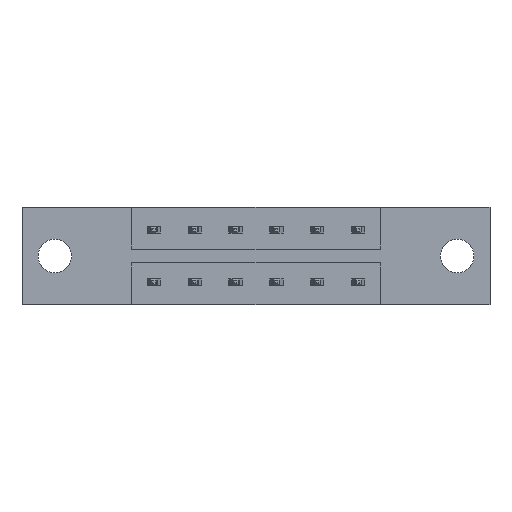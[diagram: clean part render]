
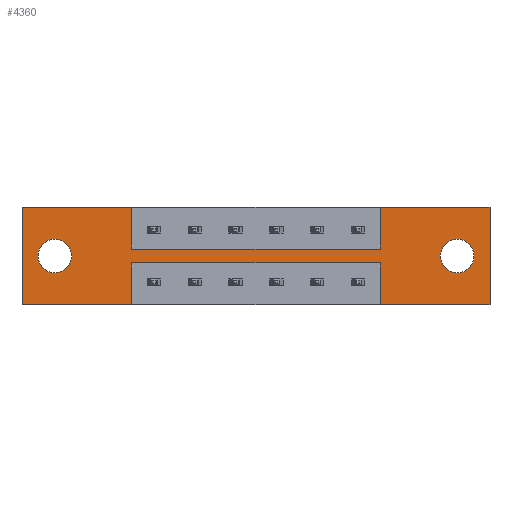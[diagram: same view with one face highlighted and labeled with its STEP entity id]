
A CAD part, front view. The second image highlights one B-rep face of the part: STEP entity #4360.
In plain terms, the highlighted planar face has unit normal (0, -1, 0).
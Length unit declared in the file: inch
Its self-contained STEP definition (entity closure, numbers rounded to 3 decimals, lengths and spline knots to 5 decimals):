
#83 = DIRECTION ( 'NONE',  ( 0., 0., 1. ) ) ;
#86 = EDGE_CURVE ( 'NONE', #4618, #5407, #849, .T. ) ;
#209 = DIRECTION ( 'NONE',  ( 0., 1., 0. ) ) ;
#345 = LINE ( 'NONE', #2995, #7201 ) ;
#614 = DIRECTION ( 'NONE',  ( 0., 1., 0. ) ) ;
#626 = CARTESIAN_POINT ( 'NONE',  ( 0., 0., -0.37 ) ) ;
#818 = EDGE_CURVE ( 'NONE', #3925, #4857, #345, .T. ) ;
#849 = CIRCLE ( 'NONE', #7057, 0.064 ) ;
#863 = EDGE_CURVE ( 'NONE', #5407, #4618, #3503, .T. ) ;
#880 = CIRCLE ( 'NONE', #7218, 0.064 ) ;
#951 = ORIENTED_EDGE ( 'NONE', *, *, #6117, .F. ) ;
#955 = FACE_OUTER_BOUND ( 'NONE', #8546, .T. ) ;
#981 = CARTESIAN_POINT ( 'NONE',  ( 1.3665, 0., -0.1585 ) ) ;
#999 = CARTESIAN_POINT ( 'NONE',  ( 1.659, 0., -0.185 ) ) ;
#1047 = CARTESIAN_POINT ( 'NONE',  ( 1.659, 0., -0.185 ) ) ;
#1057 = AXIS2_PLACEMENT_3D ( 'NONE', #626, #5760, #5850 ) ;
#1123 = CARTESIAN_POINT ( 'NONE',  ( 0.4175, 0., -0.1585 ) ) ;
#1595 = ORIENTED_EDGE ( 'NONE', *, *, #6617, .F. ) ;
#1644 = LINE ( 'NONE', #1123, #7134 ) ;
#1789 = CARTESIAN_POINT ( 'NONE',  ( 0.125, 0., -0.185 ) ) ;
#1860 = CARTESIAN_POINT ( 'NONE',  ( 0., 0., 0. ) ) ;
#1899 = EDGE_LOOP ( 'NONE', ( #1910, #5294 ) ) ;
#1910 = ORIENTED_EDGE ( 'NONE', *, *, #6625, .T. ) ;
#1950 = LINE ( 'NONE', #4713, #5332 ) ;
#2017 = CARTESIAN_POINT ( 'NONE',  ( 0.125, 0., -0.249 ) ) ;
#2071 = ORIENTED_EDGE ( 'NONE', *, *, #4004, .F. ) ;
#2097 = AXIS2_PLACEMENT_3D ( 'NONE', #8173, #209, #6837 ) ;
#2137 = CARTESIAN_POINT ( 'NONE',  ( 0.4175, 0., -0.1585 ) ) ;
#2262 = DIRECTION ( 'NONE',  ( -1., 0., 0. ) ) ;
#2313 = CIRCLE ( 'NONE', #7278, 0.064 ) ;
#2372 = LINE ( 'NONE', #7652, #5207 ) ;
#2414 = CARTESIAN_POINT ( 'NONE',  ( 1.784, 0., 0. ) ) ;
#2591 = CARTESIAN_POINT ( 'NONE',  ( 0.4175, 0., -0.37 ) ) ;
#2671 = ORIENTED_EDGE ( 'NONE', *, *, #7675, .F. ) ;
#2829 = CARTESIAN_POINT ( 'NONE',  ( 0., 0., -0.37 ) ) ;
#2886 = ORIENTED_EDGE ( 'NONE', *, *, #818, .F. ) ;
#2903 = VERTEX_POINT ( 'NONE', #3596 ) ;
#2921 = DIRECTION ( 'NONE',  ( 1., 0., 0. ) ) ;
#2995 = CARTESIAN_POINT ( 'NONE',  ( 0.4175, 0., -0.2115 ) ) ;
#3035 = LINE ( 'NONE', #5677, #3541 ) ;
#3038 = DIRECTION ( 'NONE',  ( 0., 0., 1. ) ) ;
#3078 = DIRECTION ( 'NONE',  ( 0., 0., 1. ) ) ;
#3148 = ORIENTED_EDGE ( 'NONE', *, *, #7318, .F. ) ;
#3171 = LINE ( 'NONE', #1860, #5995 ) ;
#3231 = EDGE_CURVE ( 'NONE', #3285, #6964, #4940, .T. ) ;
#3285 = VERTEX_POINT ( 'NONE', #4134 ) ;
#3381 = VECTOR ( 'NONE', #3816, 39.37008 ) ;
#3485 = CARTESIAN_POINT ( 'NONE',  ( 1.3665, 0., -0.2115 ) ) ;
#3503 = CIRCLE ( 'NONE', #2097, 0.064 ) ;
#3520 = VECTOR ( 'NONE', #8188, 39.37008 ) ;
#3541 = VECTOR ( 'NONE', #3078, 39.37008 ) ;
#3596 = CARTESIAN_POINT ( 'NONE',  ( 0., 0., 0. ) ) ;
#3776 = DIRECTION ( 'NONE',  ( 0., 0., -1. ) ) ;
#3816 = DIRECTION ( 'NONE',  ( -1., 0., 0. ) ) ;
#3856 = DIRECTION ( 'NONE',  ( 1., 0., 0. ) ) ;
#3875 = VERTEX_POINT ( 'NONE', #2414 ) ;
#3883 = CARTESIAN_POINT ( 'NONE',  ( 1.659, 0., -0.121 ) ) ;
#3925 = VERTEX_POINT ( 'NONE', #5857 ) ;
#4004 = EDGE_CURVE ( 'NONE', #2903, #3285, #3171, .T. ) ;
#4123 = VECTOR ( 'NONE', #6334, 39.37008 ) ;
#4134 = CARTESIAN_POINT ( 'NONE',  ( 0.4175, 0., 0. ) ) ;
#4242 = FACE_BOUND ( 'NONE', #8239, .T. ) ;
#4329 = DIRECTION ( 'NONE',  ( 0., 0., -1. ) ) ;
#4332 = VECTOR ( 'NONE', #2921, 39.37008 ) ;
#4360 = ADVANCED_FACE ( 'NONE', ( #5040, #4242, #955 ), #7683, .T. ) ;
#4426 = DIRECTION ( 'NONE',  ( 0., 0., 1. ) ) ;
#4618 = VERTEX_POINT ( 'NONE', #2017 ) ;
#4713 = CARTESIAN_POINT ( 'NONE',  ( 1.784, 0., 0. ) ) ;
#4715 = LINE ( 'NONE', #7917, #7510 ) ;
#4844 = DIRECTION ( 'NONE',  ( 0., 0., -1. ) ) ;
#4857 = VERTEX_POINT ( 'NONE', #2591 ) ;
#4860 = CARTESIAN_POINT ( 'NONE',  ( 1.784, 0., -0.37 ) ) ;
#4940 = LINE ( 'NONE', #2137, #3520 ) ;
#4946 = VERTEX_POINT ( 'NONE', #6655 ) ;
#4986 = VERTEX_POINT ( 'NONE', #7484 ) ;
#5038 = LINE ( 'NONE', #5673, #4123 ) ;
#5040 = FACE_BOUND ( 'NONE', #1899, .T. ) ;
#5052 = CARTESIAN_POINT ( 'NONE',  ( 0., 0., -0.37 ) ) ;
#5053 = ORIENTED_EDGE ( 'NONE', *, *, #86, .T. ) ;
#5087 = CARTESIAN_POINT ( 'NONE',  ( 1.3665, 0., 0. ) ) ;
#5207 = VECTOR ( 'NONE', #3038, 39.37008 ) ;
#5288 = EDGE_CURVE ( 'NONE', #7785, #3925, #5038, .T. ) ;
#5294 = ORIENTED_EDGE ( 'NONE', *, *, #7929, .T. ) ;
#5332 = VECTOR ( 'NONE', #8484, 39.37008 ) ;
#5407 = VERTEX_POINT ( 'NONE', #7194 ) ;
#5426 = CARTESIAN_POINT ( 'NONE',  ( 0.4175, 0., -0.1585 ) ) ;
#5507 = ORIENTED_EDGE ( 'NONE', *, *, #8329, .F. ) ;
#5657 = VERTEX_POINT ( 'NONE', #981 ) ;
#5673 = CARTESIAN_POINT ( 'NONE',  ( 0.4175, 0., -0.2115 ) ) ;
#5677 = CARTESIAN_POINT ( 'NONE',  ( 1.3665, 0., -0.2115 ) ) ;
#5760 = DIRECTION ( 'NONE',  ( 0., -1., 0. ) ) ;
#5768 = VECTOR ( 'NONE', #2262, 39.37008 ) ;
#5850 = DIRECTION ( 'NONE',  ( 0., 0., -1. ) ) ;
#5857 = CARTESIAN_POINT ( 'NONE',  ( 0.4175, 0., -0.2115 ) ) ;
#5995 = VECTOR ( 'NONE', #3856, 39.37008 ) ;
#5996 = VERTEX_POINT ( 'NONE', #4860 ) ;
#6040 = VERTEX_POINT ( 'NONE', #6753 ) ;
#6117 = EDGE_CURVE ( 'NONE', #4857, #6040, #8096, .T. ) ;
#6334 = DIRECTION ( 'NONE',  ( -1., 0., 0. ) ) ;
#6353 = EDGE_CURVE ( 'NONE', #3875, #5996, #1950, .T. ) ;
#6427 = ORIENTED_EDGE ( 'NONE', *, *, #8050, .F. ) ;
#6471 = ORIENTED_EDGE ( 'NONE', *, *, #5288, .F. ) ;
#6617 = EDGE_CURVE ( 'NONE', #5657, #6702, #2372, .T. ) ;
#6625 = EDGE_CURVE ( 'NONE', #7242, #4946, #2313, .T. ) ;
#6655 = CARTESIAN_POINT ( 'NONE',  ( 1.659, 0., -0.249 ) ) ;
#6668 = EDGE_CURVE ( 'NONE', #6964, #5657, #1644, .T. ) ;
#6702 = VERTEX_POINT ( 'NONE', #5087 ) ;
#6753 = CARTESIAN_POINT ( 'NONE',  ( 0., 0., -0.37 ) ) ;
#6837 = DIRECTION ( 'NONE',  ( 0., 0., 1. ) ) ;
#6964 = VERTEX_POINT ( 'NONE', #5426 ) ;
#7057 = AXIS2_PLACEMENT_3D ( 'NONE', #1789, #614, #4426 ) ;
#7134 = VECTOR ( 'NONE', #8345, 39.37008 ) ;
#7194 = CARTESIAN_POINT ( 'NONE',  ( 0.125, 0., -0.121 ) ) ;
#7201 = VECTOR ( 'NONE', #4844, 39.37008 ) ;
#7218 = AXIS2_PLACEMENT_3D ( 'NONE', #1047, #7694, #4329 ) ;
#7242 = VERTEX_POINT ( 'NONE', #3883 ) ;
#7278 = AXIS2_PLACEMENT_3D ( 'NONE', #999, #8381, #3776 ) ;
#7318 = EDGE_CURVE ( 'NONE', #6702, #3875, #8190, .T. ) ;
#7484 = CARTESIAN_POINT ( 'NONE',  ( 1.3665, 0., -0.37 ) ) ;
#7494 = CARTESIAN_POINT ( 'NONE',  ( 0., 0., 0. ) ) ;
#7510 = VECTOR ( 'NONE', #83, 39.37008 ) ;
#7542 = ORIENTED_EDGE ( 'NONE', *, *, #863, .T. ) ;
#7652 = CARTESIAN_POINT ( 'NONE',  ( 1.3665, 0., -0.1585 ) ) ;
#7675 = EDGE_CURVE ( 'NONE', #6040, #2903, #4715, .T. ) ;
#7683 = PLANE ( 'NONE',  #1057 ) ;
#7694 = DIRECTION ( 'NONE',  ( 0., 1., 0. ) ) ;
#7698 = ORIENTED_EDGE ( 'NONE', *, *, #6353, .F. ) ;
#7778 = ORIENTED_EDGE ( 'NONE', *, *, #3231, .F. ) ;
#7782 = LINE ( 'NONE', #5052, #3381 ) ;
#7785 = VERTEX_POINT ( 'NONE', #3485 ) ;
#7917 = CARTESIAN_POINT ( 'NONE',  ( 0., 0., 0. ) ) ;
#7929 = EDGE_CURVE ( 'NONE', #4946, #7242, #880, .T. ) ;
#8050 = EDGE_CURVE ( 'NONE', #5996, #4986, #7782, .T. ) ;
#8096 = LINE ( 'NONE', #2829, #5768 ) ;
#8173 = CARTESIAN_POINT ( 'NONE',  ( 0.125, 0., -0.185 ) ) ;
#8188 = DIRECTION ( 'NONE',  ( 0., 0., -1. ) ) ;
#8190 = LINE ( 'NONE', #7494, #4332 ) ;
#8239 = EDGE_LOOP ( 'NONE', ( #7542, #5053 ) ) ;
#8329 = EDGE_CURVE ( 'NONE', #4986, #7785, #3035, .T. ) ;
#8345 = DIRECTION ( 'NONE',  ( 1., 0., 0. ) ) ;
#8381 = DIRECTION ( 'NONE',  ( 0., 1., 0. ) ) ;
#8430 = ORIENTED_EDGE ( 'NONE', *, *, #6668, .F. ) ;
#8484 = DIRECTION ( 'NONE',  ( 0., 0., -1. ) ) ;
#8546 = EDGE_LOOP ( 'NONE', ( #5507, #6427, #7698, #3148, #1595, #8430, #7778, #2071, #2671, #951, #2886, #6471 ) ) ;
